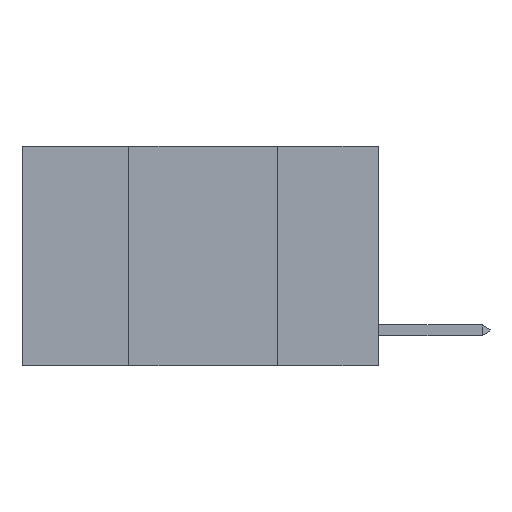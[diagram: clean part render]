
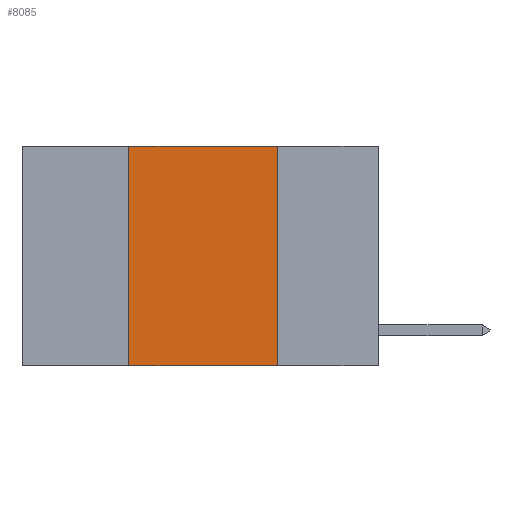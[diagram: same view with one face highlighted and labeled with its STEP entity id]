
A CAD part, left-side view. The second image highlights one B-rep face of the part: STEP entity #8085.
In plain terms, the highlighted planar face has unit normal (-1, 0, 0).
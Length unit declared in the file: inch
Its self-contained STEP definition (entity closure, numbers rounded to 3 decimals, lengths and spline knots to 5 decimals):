
#758 = VECTOR ( 'NONE', #9599, 39.37008 ) ;
#776 = DIRECTION ( 'NONE',  ( 0., 0., -1. ) ) ;
#859 = CARTESIAN_POINT ( 'NONE',  ( 0., 0.42, 0. ) ) ;
#1018 = ORIENTED_EDGE ( 'NONE', *, *, #6677, .F. ) ;
#1093 = EDGE_CURVE ( 'NONE', #11616, #12713, #2175, .T. ) ;
#1235 = ORIENTED_EDGE ( 'NONE', *, *, #1093, .F. ) ;
#1872 = CARTESIAN_POINT ( 'NONE',  ( 0., 0.17, 0. ) ) ;
#2076 = EDGE_CURVE ( 'NONE', #4907, #5966, #4932, .T. ) ;
#2175 = LINE ( 'NONE', #12564, #8271 ) ;
#2289 = ORIENTED_EDGE ( 'NONE', *, *, #2076, .F. ) ;
#2649 = LINE ( 'NONE', #10033, #9058 ) ;
#3355 = EDGE_LOOP ( 'NONE', ( #2289, #1018, #1235, #11031 ) ) ;
#3462 = LINE ( 'NONE', #3708, #758 ) ;
#3708 = CARTESIAN_POINT ( 'NONE',  ( 0., 0.6, -0.37 ) ) ;
#4065 = DIRECTION ( 'NONE',  ( 0., 0., -1. ) ) ;
#4654 = DIRECTION ( 'NONE',  ( 0., 0., 1. ) ) ;
#4907 = VERTEX_POINT ( 'NONE', #11477 ) ;
#4932 = LINE ( 'NONE', #1872, #9089 ) ;
#5287 = CARTESIAN_POINT ( 'NONE',  ( 0., 0.17, -0.37 ) ) ;
#5966 = VERTEX_POINT ( 'NONE', #5287 ) ;
#6677 = EDGE_CURVE ( 'NONE', #12713, #4907, #2649, .T. ) ;
#7015 = DIRECTION ( 'NONE',  ( 0., -1., 0. ) ) ;
#7673 = FACE_OUTER_BOUND ( 'NONE', #3355, .T. ) ;
#8085 = ADVANCED_FACE ( 'NONE', ( #7673 ), #10499, .F. ) ;
#8135 = CARTESIAN_POINT ( 'NONE',  ( 0., 0.42, -0.37 ) ) ;
#8271 = VECTOR ( 'NONE', #4654, 39.37008 ) ;
#9058 = VECTOR ( 'NONE', #7015, 39.37008 ) ;
#9089 = VECTOR ( 'NONE', #4065, 39.37008 ) ;
#9599 = DIRECTION ( 'NONE',  ( 0., -1., 0. ) ) ;
#10033 = CARTESIAN_POINT ( 'NONE',  ( 0., 0.6, 0. ) ) ;
#10119 = AXIS2_PLACEMENT_3D ( 'NONE', #12408, #11583, #776 ) ;
#10411 = EDGE_CURVE ( 'NONE', #11616, #5966, #3462, .T. ) ;
#10499 = PLANE ( 'NONE',  #10119 ) ;
#11031 = ORIENTED_EDGE ( 'NONE', *, *, #10411, .T. ) ;
#11477 = CARTESIAN_POINT ( 'NONE',  ( 0., 0.17, 0. ) ) ;
#11583 = DIRECTION ( 'NONE',  ( 1., 0., 0. ) ) ;
#11616 = VERTEX_POINT ( 'NONE', #8135 ) ;
#12408 = CARTESIAN_POINT ( 'NONE',  ( 0., 0.6, 0. ) ) ;
#12564 = CARTESIAN_POINT ( 'NONE',  ( 0., 0.42, 0. ) ) ;
#12713 = VERTEX_POINT ( 'NONE', #859 ) ;
